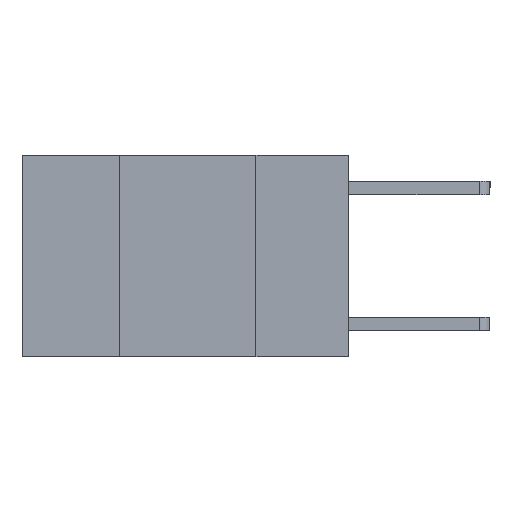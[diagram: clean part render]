
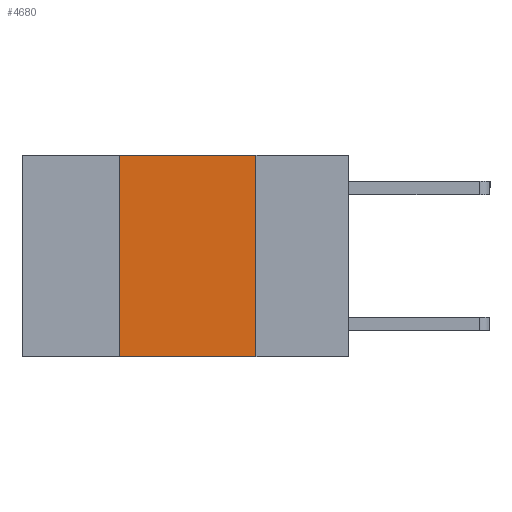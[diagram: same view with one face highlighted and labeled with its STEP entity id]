
A CAD part, left-side view. The second image highlights one B-rep face of the part: STEP entity #4680.
In plain terms, the highlighted planar face has unit normal (-1, 0, 0).
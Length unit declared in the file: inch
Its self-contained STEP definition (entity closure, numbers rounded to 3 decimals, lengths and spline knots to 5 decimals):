
#76 = CARTESIAN_POINT ( 'NONE',  ( 0., 0.42, 0. ) ) ;
#274 = VECTOR ( 'NONE', #4000, 39.37008 ) ;
#597 = EDGE_CURVE ( 'NONE', #3575, #7308, #9660, .T. ) ;
#1133 = EDGE_LOOP ( 'NONE', ( #10743, #3175, #3305, #8612 ) ) ;
#1283 = DIRECTION ( 'NONE',  ( 0., 0., -1. ) ) ;
#1674 = PLANE ( 'NONE',  #9690 ) ;
#1724 = CARTESIAN_POINT ( 'NONE',  ( 0., 0.17, 0. ) ) ;
#1834 = CARTESIAN_POINT ( 'NONE',  ( 0., 0.17, 0. ) ) ;
#2422 = DIRECTION ( 'NONE',  ( 1., 0., 0. ) ) ;
#2536 = EDGE_CURVE ( 'NONE', #4472, #3575, #9357, .T. ) ;
#2600 = CARTESIAN_POINT ( 'NONE',  ( 0., 0.42, 0. ) ) ;
#2963 = EDGE_CURVE ( 'NONE', #3540, #7308, #6882, .T. ) ;
#3175 = ORIENTED_EDGE ( 'NONE', *, *, #2536, .F. ) ;
#3212 = CARTESIAN_POINT ( 'NONE',  ( 0., 0.17, -0.37 ) ) ;
#3305 = ORIENTED_EDGE ( 'NONE', *, *, #4890, .F. ) ;
#3540 = VERTEX_POINT ( 'NONE', #10573 ) ;
#3575 = VERTEX_POINT ( 'NONE', #1834 ) ;
#4000 = DIRECTION ( 'NONE',  ( 0., 0., 1. ) ) ;
#4161 = CARTESIAN_POINT ( 'NONE',  ( 0., 0.6, 0. ) ) ;
#4203 = VECTOR ( 'NONE', #7650, 39.37008 ) ;
#4472 = VERTEX_POINT ( 'NONE', #76 ) ;
#4680 = ADVANCED_FACE ( 'NONE', ( #5718 ), #1674, .F. ) ;
#4890 = EDGE_CURVE ( 'NONE', #3540, #4472, #10532, .T. ) ;
#5299 = DIRECTION ( 'NONE',  ( 0., 0., -1. ) ) ;
#5718 = FACE_OUTER_BOUND ( 'NONE', #1133, .T. ) ;
#5945 = CARTESIAN_POINT ( 'NONE',  ( 0., 0.6, -0.37 ) ) ;
#6650 = VECTOR ( 'NONE', #10363, 39.37008 ) ;
#6882 = LINE ( 'NONE', #5945, #6650 ) ;
#7308 = VERTEX_POINT ( 'NONE', #3212 ) ;
#7650 = DIRECTION ( 'NONE',  ( 0., -1., 0. ) ) ;
#8612 = ORIENTED_EDGE ( 'NONE', *, *, #2963, .T. ) ;
#9357 = LINE ( 'NONE', #4161, #4203 ) ;
#9660 = LINE ( 'NONE', #1724, #10643 ) ;
#9690 = AXIS2_PLACEMENT_3D ( 'NONE', #10412, #2422, #1283 ) ;
#10363 = DIRECTION ( 'NONE',  ( 0., -1., 0. ) ) ;
#10412 = CARTESIAN_POINT ( 'NONE',  ( 0., 0.6, 0. ) ) ;
#10532 = LINE ( 'NONE', #2600, #274 ) ;
#10573 = CARTESIAN_POINT ( 'NONE',  ( 0., 0.42, -0.37 ) ) ;
#10643 = VECTOR ( 'NONE', #5299, 39.37008 ) ;
#10743 = ORIENTED_EDGE ( 'NONE', *, *, #597, .F. ) ;
